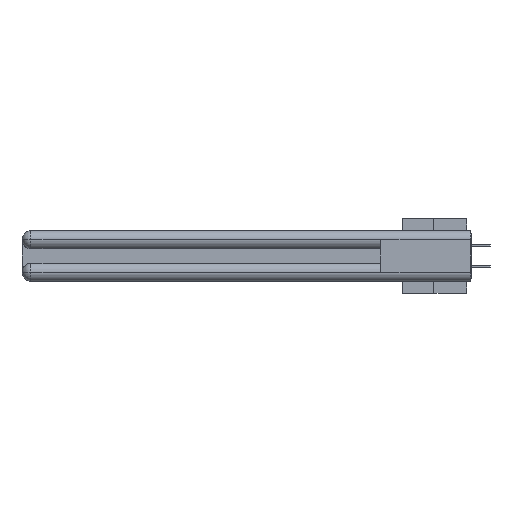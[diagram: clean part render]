
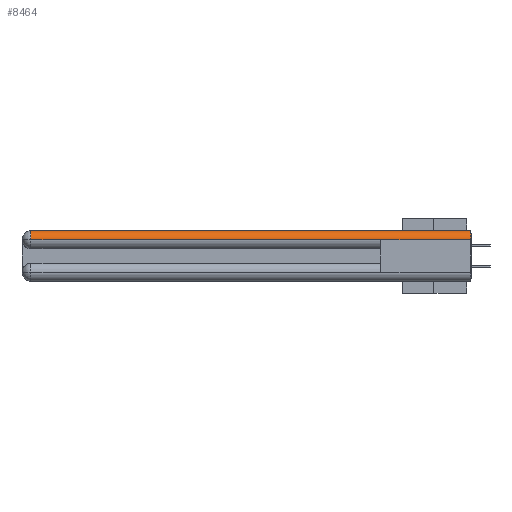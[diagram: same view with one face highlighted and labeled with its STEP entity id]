
A CAD part, left-side view. The second image highlights one B-rep face of the part: STEP entity #8464.
In plain terms, the highlighted cylindrical face has radius 1.562 mm (diameter 3.124 mm), a partial arc.
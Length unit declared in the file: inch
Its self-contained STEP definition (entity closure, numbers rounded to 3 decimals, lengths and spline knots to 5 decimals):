
#2126 = DIRECTION ( 'NONE',  ( 0., 1., 0. ) ) ;
#2940 = CARTESIAN_POINT ( 'NONE',  ( 0.0615, 0., 0. ) ) ;
#3041 = FACE_OUTER_BOUND ( 'NONE', #31534, .T. ) ;
#3939 = EDGE_CURVE ( 'NONE', #18014, #17600, #41480, .T. ) ;
#4420 = EDGE_CURVE ( 'NONE', #30576, #17600, #25009, .T. ) ;
#4546 = AXIS2_PLACEMENT_3D ( 'NONE', #45876, #31732, #16988 ) ;
#6252 = DIRECTION ( 'NONE',  ( 0., 0., 1. ) ) ;
#6255 = ORIENTED_EDGE ( 'NONE', *, *, #4420, .T. ) ;
#7163 = CARTESIAN_POINT ( 'NONE',  ( 0., 3., -0.0615 ) ) ;
#8015 = ORIENTED_EDGE ( 'NONE', *, *, #40366, .F. ) ;
#8464 = ADVANCED_FACE ( 'NONE', ( #3041 ), #16127, .T. ) ;
#8750 = AXIS2_PLACEMENT_3D ( 'NONE', #14149, #12029, #6252 ) ;
#10249 = EDGE_CURVE ( 'NONE', #31121, #30576, #12567, .T. ) ;
#10674 = DIRECTION ( 'NONE',  ( 1., 0., 0. ) ) ;
#12029 = DIRECTION ( 'NONE',  ( 0., 1., 0. ) ) ;
#12567 = CIRCLE ( 'NONE', #4546, 0.0615 ) ;
#12933 = DIRECTION ( 'NONE',  ( 0., -1., 0. ) ) ;
#14149 = CARTESIAN_POINT ( 'NONE',  ( 0.0615, 0., -0.0615 ) ) ;
#14584 = DIRECTION ( 'NONE',  ( 0., -1., 0. ) ) ;
#16127 = CYLINDRICAL_SURFACE ( 'NONE', #8750, 0.0615 ) ;
#16988 = DIRECTION ( 'NONE',  ( 0., 0., 1. ) ) ;
#17600 = VERTEX_POINT ( 'NONE', #19489 ) ;
#18014 = VERTEX_POINT ( 'NONE', #39066 ) ;
#18706 = CARTESIAN_POINT ( 'NONE',  ( 0.0615, 2.94, 0. ) ) ;
#18765 = CARTESIAN_POINT ( 'NONE',  ( 0., 2.94, -0.0615 ) ) ;
#19489 = CARTESIAN_POINT ( 'NONE',  ( 0., 0.6, -0.0615 ) ) ;
#21815 = ORIENTED_EDGE ( 'NONE', *, *, #39044, .F. ) ;
#22308 = ORIENTED_EDGE ( 'NONE', *, *, #10249, .T. ) ;
#22738 = VERTEX_POINT ( 'NONE', #2940 ) ;
#25009 = LINE ( 'NONE', #7163, #44867 ) ;
#27520 = CARTESIAN_POINT ( 'NONE',  ( 0., 3., -0.0615 ) ) ;
#28728 = DIRECTION ( 'NONE',  ( 0., -1., 0. ) ) ;
#29051 = CARTESIAN_POINT ( 'NONE',  ( 0.0615, 0., -0.0615 ) ) ;
#30174 = VECTOR ( 'NONE', #12933, 39.37008 ) ;
#30576 = VERTEX_POINT ( 'NONE', #18765 ) ;
#31121 = VERTEX_POINT ( 'NONE', #18706 ) ;
#31534 = EDGE_LOOP ( 'NONE', ( #8015, #22308, #6255, #41444, #21815 ) ) ;
#31732 = DIRECTION ( 'NONE',  ( 0., -1., 0. ) ) ;
#33305 = CIRCLE ( 'NONE', #39726, 0.0615 ) ;
#38117 = LINE ( 'NONE', #42116, #30174 ) ;
#39044 = EDGE_CURVE ( 'NONE', #22738, #18014, #33305, .T. ) ;
#39066 = CARTESIAN_POINT ( 'NONE',  ( 0., 0., -0.0615 ) ) ;
#39726 = AXIS2_PLACEMENT_3D ( 'NONE', #29051, #28728, #10674 ) ;
#40366 = EDGE_CURVE ( 'NONE', #31121, #22738, #38117, .T. ) ;
#41444 = ORIENTED_EDGE ( 'NONE', *, *, #3939, .F. ) ;
#41480 = LINE ( 'NONE', #27520, #43215 ) ;
#42116 = CARTESIAN_POINT ( 'NONE',  ( 0.0615, 0., 0. ) ) ;
#43215 = VECTOR ( 'NONE', #2126, 39.37008 ) ;
#44867 = VECTOR ( 'NONE', #14584, 39.37008 ) ;
#45876 = CARTESIAN_POINT ( 'NONE',  ( 0.0615, 2.94, -0.0615 ) ) ;
